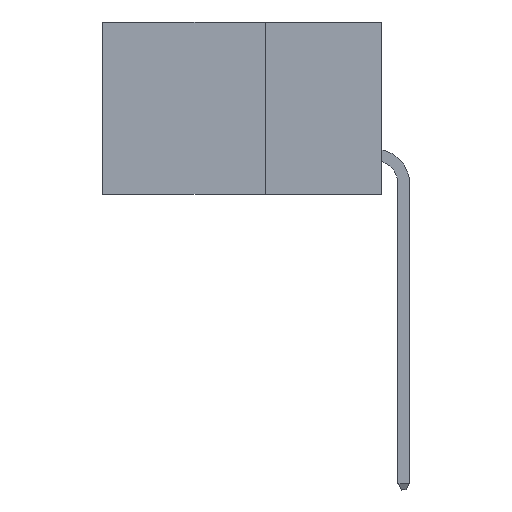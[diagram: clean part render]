
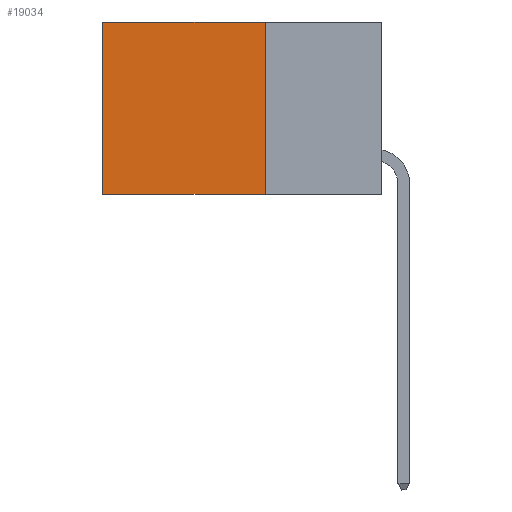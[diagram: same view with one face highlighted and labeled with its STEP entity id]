
A CAD part, left-side view. The second image highlights one B-rep face of the part: STEP entity #19034.
In plain terms, the highlighted planar face has unit normal (-1, 0, 0).
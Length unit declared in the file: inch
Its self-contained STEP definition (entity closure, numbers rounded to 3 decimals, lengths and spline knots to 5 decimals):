
#212 = DIRECTION ( 'NONE',  ( 0., 0., -1. ) ) ;
#838 = VECTOR ( 'NONE', #14615, 39.37008 ) ;
#1309 = EDGE_CURVE ( 'NONE', #16167, #5158, #22220, .T. ) ;
#1718 = EDGE_CURVE ( 'NONE', #21425, #16167, #7243, .T. ) ;
#2405 = EDGE_LOOP ( 'NONE', ( #17385, #22793, #18599, #21208 ) ) ;
#2799 = EDGE_CURVE ( 'NONE', #15270, #5158, #11544, .T. ) ;
#2948 = DIRECTION ( 'NONE',  ( 0., 0., -1. ) ) ;
#5064 = DIRECTION ( 'NONE',  ( 0., 1., 0. ) ) ;
#5158 = VERTEX_POINT ( 'NONE', #11322 ) ;
#5786 = AXIS2_PLACEMENT_3D ( 'NONE', #12249, #18045, #2948 ) ;
#6437 = CARTESIAN_POINT ( 'NONE',  ( 0.2875, 0.25, 0. ) ) ;
#7230 = CARTESIAN_POINT ( 'NONE',  ( 0.2875, 0.25, 0. ) ) ;
#7243 = LINE ( 'NONE', #11248, #838 ) ;
#10692 = CARTESIAN_POINT ( 'NONE',  ( 0.2875, 0.25, -0.37 ) ) ;
#11018 = CARTESIAN_POINT ( 'NONE',  ( 0.2875, 0.25, -0.37 ) ) ;
#11248 = CARTESIAN_POINT ( 'NONE',  ( 0.2875, 0.25, 0. ) ) ;
#11322 = CARTESIAN_POINT ( 'NONE',  ( 0.2875, 0.6, -0.37 ) ) ;
#11544 = LINE ( 'NONE', #19194, #19661 ) ;
#12249 = CARTESIAN_POINT ( 'NONE',  ( 0.2875, 0.25, 0. ) ) ;
#13191 = EDGE_CURVE ( 'NONE', #21425, #15270, #24394, .T. ) ;
#14615 = DIRECTION ( 'NONE',  ( 0., 0., -1. ) ) ;
#15270 = VERTEX_POINT ( 'NONE', #21714 ) ;
#15596 = VECTOR ( 'NONE', #20382, 39.37008 ) ;
#16167 = VERTEX_POINT ( 'NONE', #11018 ) ;
#17385 = ORIENTED_EDGE ( 'NONE', *, *, #2799, .T. ) ;
#18045 = DIRECTION ( 'NONE',  ( 1., 0., 0. ) ) ;
#18599 = ORIENTED_EDGE ( 'NONE', *, *, #1718, .F. ) ;
#19034 = ADVANCED_FACE ( 'NONE', ( #21806 ), #19920, .F. ) ;
#19161 = VECTOR ( 'NONE', #5064, 39.37008 ) ;
#19194 = CARTESIAN_POINT ( 'NONE',  ( 0.2875, 0.6, 0. ) ) ;
#19661 = VECTOR ( 'NONE', #212, 39.37008 ) ;
#19920 = PLANE ( 'NONE',  #5786 ) ;
#20382 = DIRECTION ( 'NONE',  ( 0., 1., 0. ) ) ;
#21208 = ORIENTED_EDGE ( 'NONE', *, *, #13191, .T. ) ;
#21425 = VERTEX_POINT ( 'NONE', #6437 ) ;
#21714 = CARTESIAN_POINT ( 'NONE',  ( 0.2875, 0.6, 0. ) ) ;
#21806 = FACE_OUTER_BOUND ( 'NONE', #2405, .T. ) ;
#22220 = LINE ( 'NONE', #10692, #19161 ) ;
#22793 = ORIENTED_EDGE ( 'NONE', *, *, #1309, .F. ) ;
#24394 = LINE ( 'NONE', #7230, #15596 ) ;
